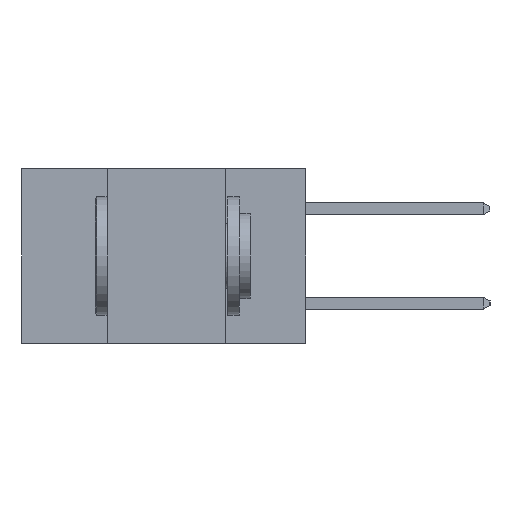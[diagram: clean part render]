
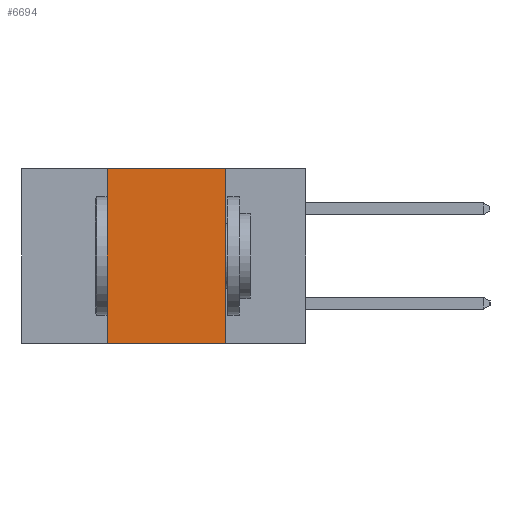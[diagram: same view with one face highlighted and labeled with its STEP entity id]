
A CAD part, left-side view. The second image highlights one B-rep face of the part: STEP entity #6694.
In plain terms, the highlighted planar face has unit normal (-1, 0, 0).
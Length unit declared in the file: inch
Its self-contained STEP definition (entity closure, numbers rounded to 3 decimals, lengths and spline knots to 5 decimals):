
#64 = CARTESIAN_POINT ( 'NONE',  ( 0., 0.17, 0. ) ) ;
#730 = ORIENTED_EDGE ( 'NONE', *, *, #16915, .F. ) ;
#858 = LINE ( 'NONE', #3025, #8885 ) ;
#1032 = DIRECTION ( 'NONE',  ( 0., 0., -1. ) ) ;
#1233 = DIRECTION ( 'NONE',  ( 1., 0., 0. ) ) ;
#1279 = PLANE ( 'NONE',  #5818 ) ;
#1740 = CARTESIAN_POINT ( 'NONE',  ( 0., 0.6, 0. ) ) ;
#2676 = ORIENTED_EDGE ( 'NONE', *, *, #15023, .T. ) ;
#2981 = CARTESIAN_POINT ( 'NONE',  ( 0., 0.42, 0. ) ) ;
#3025 = CARTESIAN_POINT ( 'NONE',  ( 0., 0.6, 0. ) ) ;
#3495 = EDGE_LOOP ( 'NONE', ( #8332, #10787, #730, #2676 ) ) ;
#5818 = AXIS2_PLACEMENT_3D ( 'NONE', #1740, #1233, #1032 ) ;
#6057 = VECTOR ( 'NONE', #8875, 39.37008 ) ;
#6300 = VERTEX_POINT ( 'NONE', #64 ) ;
#6694 = ADVANCED_FACE ( 'NONE', ( #18320 ), #1279, .F. ) ;
#6789 = CARTESIAN_POINT ( 'NONE',  ( 0., 0.17, -0.37 ) ) ;
#8332 = ORIENTED_EDGE ( 'NONE', *, *, #18507, .F. ) ;
#8875 = DIRECTION ( 'NONE',  ( 0., 0., -1. ) ) ;
#8885 = VECTOR ( 'NONE', #13349, 39.37008 ) ;
#8991 = CARTESIAN_POINT ( 'NONE',  ( 0., 0.42, -0.37 ) ) ;
#10377 = CARTESIAN_POINT ( 'NONE',  ( 0., 0.6, -0.37 ) ) ;
#10458 = VECTOR ( 'NONE', #13590, 39.37008 ) ;
#10787 = ORIENTED_EDGE ( 'NONE', *, *, #17898, .F. ) ;
#11408 = VERTEX_POINT ( 'NONE', #8991 ) ;
#12114 = CARTESIAN_POINT ( 'NONE',  ( 0., 0.42, -0.37 ) ) ;
#12762 = VECTOR ( 'NONE', #14785, 39.37008 ) ;
#13349 = DIRECTION ( 'NONE',  ( 0., -1., 0. ) ) ;
#13590 = DIRECTION ( 'NONE',  ( 0., 0., 1. ) ) ;
#13673 = LINE ( 'NONE', #10377, #12762 ) ;
#14785 = DIRECTION ( 'NONE',  ( 0., -1., 0. ) ) ;
#15023 = EDGE_CURVE ( 'NONE', #11408, #17209, #13673, .T. ) ;
#16915 = EDGE_CURVE ( 'NONE', #11408, #17509, #18613, .T. ) ;
#17209 = VERTEX_POINT ( 'NONE', #6789 ) ;
#17214 = LINE ( 'NONE', #17536, #6057 ) ;
#17509 = VERTEX_POINT ( 'NONE', #2981 ) ;
#17536 = CARTESIAN_POINT ( 'NONE',  ( 0., 0.17, -0.37 ) ) ;
#17898 = EDGE_CURVE ( 'NONE', #17509, #6300, #858, .T. ) ;
#18320 = FACE_OUTER_BOUND ( 'NONE', #3495, .T. ) ;
#18507 = EDGE_CURVE ( 'NONE', #6300, #17209, #17214, .T. ) ;
#18613 = LINE ( 'NONE', #12114, #10458 ) ;
